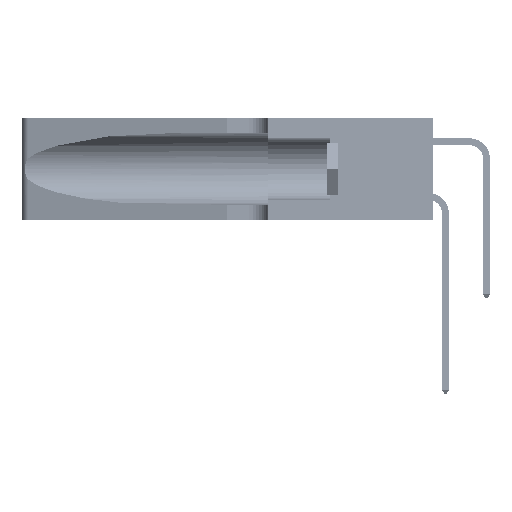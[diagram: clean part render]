
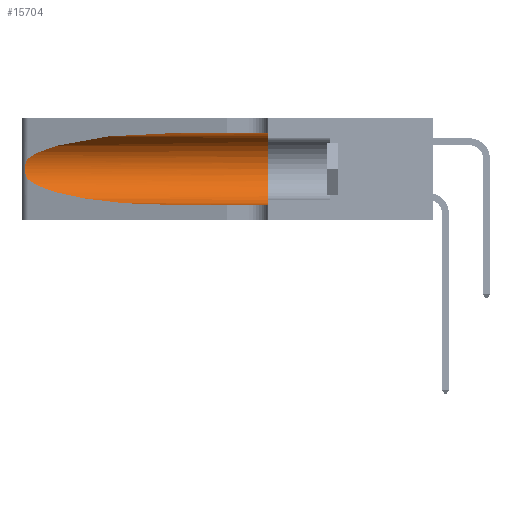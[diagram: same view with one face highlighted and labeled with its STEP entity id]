
A CAD part, left-side view. The second image highlights one B-rep face of the part: STEP entity #15704.
In plain terms, the highlighted cylindrical face has radius 3.308 mm (diameter 6.617 mm), a partial arc.
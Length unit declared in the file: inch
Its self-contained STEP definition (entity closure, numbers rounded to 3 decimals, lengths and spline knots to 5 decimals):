
#69 = CARTESIAN_POINT ( 'NONE',  ( 0.1305, 0.72297, 0.05475 ) ) ;
#621 = LINE ( 'NONE', #10718, #54338 ) ;
#768 = CARTESIAN_POINT ( 'NONE',  ( 0.1305, 0.35, 0.05475 ) ) ;
#1587 = ORIENTED_EDGE ( 'NONE', *, *, #27008, .F. ) ;
#2345 = DIRECTION ( 'NONE',  ( 0., 0., 1. ) ) ;
#2696 = CARTESIAN_POINT ( 'NONE',  ( 0.26018, 1.23835, 0.19895 ) ) ;
#4064 = CARTESIAN_POINT ( 'NONE',  ( 0.25487, 1.22718, 0.22369 ) ) ;
#4315 = EDGE_LOOP ( 'NONE', ( #21437, #48759, #35268, #12891, #14787, #1587 ) ) ;
#5168 = CARTESIAN_POINT ( 'NONE',  ( 0.1305, 0.72297, 0.31525 ) ) ;
#5347 = VERTEX_POINT ( 'NONE', #34628 ) ;
#6305 = DIRECTION ( 'NONE',  ( 0., -1., 0. ) ) ;
#7088 = CARTESIAN_POINT ( 'NONE',  ( 0.26075, 1.23896, 0.178 ) ) ;
#8394 = EDGE_CURVE ( 'NONE', #35220, #51001, #51966, .T. ) ;
#10718 = CARTESIAN_POINT ( 'NONE',  ( 0.1305, 1.61858, 0.05475 ) ) ;
#11492 = CARTESIAN_POINT ( 'NONE',  ( 0.25856, 1.23593, 0.16098 ) ) ;
#12891 = ORIENTED_EDGE ( 'NONE', *, *, #16725, .T. ) ;
#13219 =( BOUNDED_CURVE ( )  B_SPLINE_CURVE ( 3, ( #56042, #47344, #34317, #4064 ),
 .UNSPECIFIED., .F., .F. ) 
 B_SPLINE_CURVE_WITH_KNOTS ( ( 4, 4 ),
 ( 1.5708, 2.84003 ),
 .UNSPECIFIED. ) 
 CURVE ( )  GEOMETRIC_REPRESENTATION_ITEM ( )  RATIONAL_B_SPLINE_CURVE ( ( 1., 0.87, 0.87, 1. ) ) 
 REPRESENTATION_ITEM ( '' )  );
#14364 = CARTESIAN_POINT ( 'NONE',  ( 0.1305, 0.72297, 0.05475 ) ) ;
#14571 = EDGE_CURVE ( 'NONE', #24458, #20044, #13219, .T. ) ;
#14787 = ORIENTED_EDGE ( 'NONE', *, *, #8394, .F. ) ;
#15704 = ADVANCED_FACE ( 'NONE', ( #26695 ), #36895, .F. ) ;
#15707 = CARTESIAN_POINT ( 'NONE',  ( 0.25555, 1.22994, 0.2215 ) ) ;
#15891 = CARTESIAN_POINT ( 'NONE',  ( 0.25639, 1.23186, 0.15144 ) ) ;
#16725 = EDGE_CURVE ( 'NONE', #45833, #51001, #621, .T. ) ;
#18553 = VECTOR ( 'NONE', #24322, 39.37008 ) ;
#19178 =( BOUNDED_CURVE ( )  B_SPLINE_CURVE ( 3, ( #40179, #31662, #40358, #14364 ),
 .UNSPECIFIED., .F., .F. ) 
 B_SPLINE_CURVE_WITH_KNOTS ( ( 4, 4 ),
 ( 3.44316, 4.71239 ),
 .UNSPECIFIED. ) 
 CURVE ( )  GEOMETRIC_REPRESENTATION_ITEM ( )  RATIONAL_B_SPLINE_CURVE ( ( 1., 0.87, 0.87, 1. ) ) 
 REPRESENTATION_ITEM ( '' )  );
#20044 = VERTEX_POINT ( 'NONE', #48186 ) ;
#20262 = CARTESIAN_POINT ( 'NONE',  ( 0.25487, 1.22718, 0.14631 ) ) ;
#21437 = ORIENTED_EDGE ( 'NONE', *, *, #14571, .T. ) ;
#24322 = DIRECTION ( 'NONE',  ( 0., -1., 0. ) ) ;
#24445 = CARTESIAN_POINT ( 'NONE',  ( 0.25639, 1.23184, 0.21858 ) ) ;
#24458 = VERTEX_POINT ( 'NONE', #5168 ) ;
#25113 = B_SPLINE_CURVE_WITH_KNOTS ( 'NONE', 3,
 ( #46035, #15707, #24445, #54700, #28782, #2696, #33147, #7088, #37518, #11492, #41868, #15891, #46220, #20262 ),
 .UNSPECIFIED., .F., .F.,
 ( 4, 2, 2, 2, 2, 2, 4 ),
 ( 0., 0.00027, 0.00053, 0.00107, 0.0016, 0.00187, 0.00214 ),
 .UNSPECIFIED. ) ;
#26695 = FACE_OUTER_BOUND ( 'NONE', #4315, .T. ) ;
#27008 = EDGE_CURVE ( 'NONE', #24458, #35220, #40274, .T. ) ;
#27542 = EDGE_CURVE ( 'NONE', #5347, #45833, #19178, .T. ) ;
#28461 = DIRECTION ( 'NONE',  ( 0., 1., 0. ) ) ;
#28678 = DIRECTION ( 'NONE',  ( 0., 0., -1. ) ) ;
#28782 = CARTESIAN_POINT ( 'NONE',  ( 0.25854, 1.2359, 0.20912 ) ) ;
#31662 = CARTESIAN_POINT ( 'NONE',  ( 0.2373, 1.15595, 0.08982 ) ) ;
#33147 = CARTESIAN_POINT ( 'NONE',  ( 0.26075, 1.23896, 0.19203 ) ) ;
#34317 = CARTESIAN_POINT ( 'NONE',  ( 0.2373, 1.15595, 0.28018 ) ) ;
#34628 = CARTESIAN_POINT ( 'NONE',  ( 0.25487, 1.22718, 0.14631 ) ) ;
#35220 = VERTEX_POINT ( 'NONE', #50644 ) ;
#35268 = ORIENTED_EDGE ( 'NONE', *, *, #27542, .T. ) ;
#36895 = CYLINDRICAL_SURFACE ( 'NONE', #40630, 0.13025 ) ;
#37518 = CARTESIAN_POINT ( 'NONE',  ( 0.26017, 1.23833, 0.17102 ) ) ;
#39175 = EDGE_CURVE ( 'NONE', #20044, #5347, #25113, .T. ) ;
#40179 = CARTESIAN_POINT ( 'NONE',  ( 0.25487, 1.22718, 0.14631 ) ) ;
#40274 = LINE ( 'NONE', #45917, #18553 ) ;
#40358 = CARTESIAN_POINT ( 'NONE',  ( 0.18966, 0.96281, 0.05475 ) ) ;
#40630 = AXIS2_PLACEMENT_3D ( 'NONE', #50438, #54776, #28678 ) ;
#41868 = CARTESIAN_POINT ( 'NONE',  ( 0.25789, 1.23486, 0.15765 ) ) ;
#42981 = AXIS2_PLACEMENT_3D ( 'NONE', #54371, #28461, #2345 ) ;
#45833 = VERTEX_POINT ( 'NONE', #69 ) ;
#45917 = CARTESIAN_POINT ( 'NONE',  ( 0.1305, 1.61858, 0.31525 ) ) ;
#46035 = CARTESIAN_POINT ( 'NONE',  ( 0.25487, 1.22718, 0.22369 ) ) ;
#46220 = CARTESIAN_POINT ( 'NONE',  ( 0.25555, 1.22993, 0.14849 ) ) ;
#47344 = CARTESIAN_POINT ( 'NONE',  ( 0.18966, 0.96281, 0.31525 ) ) ;
#48186 = CARTESIAN_POINT ( 'NONE',  ( 0.25487, 1.22718, 0.22369 ) ) ;
#48759 = ORIENTED_EDGE ( 'NONE', *, *, #39175, .T. ) ;
#50438 = CARTESIAN_POINT ( 'NONE',  ( 0.1305, 1.61858, 0.185 ) ) ;
#50644 = CARTESIAN_POINT ( 'NONE',  ( 0.1305, 0.35, 0.31525 ) ) ;
#51001 = VERTEX_POINT ( 'NONE', #768 ) ;
#51966 = CIRCLE ( 'NONE', #42981, 0.13025 ) ;
#54338 = VECTOR ( 'NONE', #6305, 39.37008 ) ;
#54371 = CARTESIAN_POINT ( 'NONE',  ( 0.1305, 0.35, 0.185 ) ) ;
#54700 = CARTESIAN_POINT ( 'NONE',  ( 0.25787, 1.23484, 0.2124 ) ) ;
#54776 = DIRECTION ( 'NONE',  ( 0., -1., 0. ) ) ;
#56042 = CARTESIAN_POINT ( 'NONE',  ( 0.1305, 0.72297, 0.31525 ) ) ;
